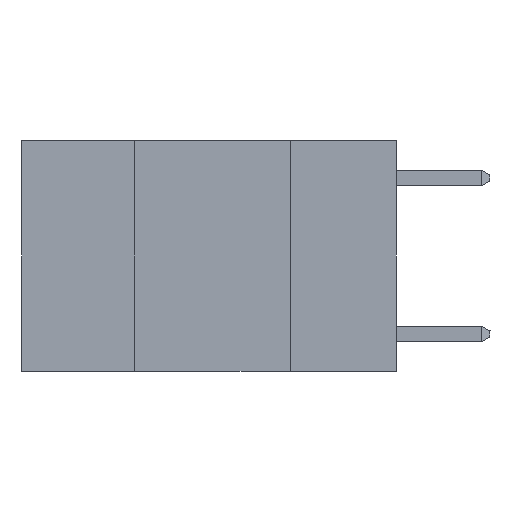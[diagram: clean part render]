
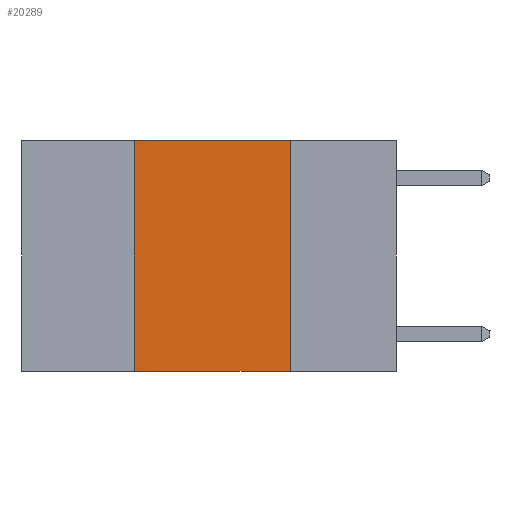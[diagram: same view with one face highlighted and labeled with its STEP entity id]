
A CAD part, left-side view. The second image highlights one B-rep face of the part: STEP entity #20289.
In plain terms, the highlighted planar face has unit normal (-1, 0, 0).
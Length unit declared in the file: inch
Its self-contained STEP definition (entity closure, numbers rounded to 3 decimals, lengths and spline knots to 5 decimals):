
#103 = VERTEX_POINT ( 'NONE', #12100 ) ;
#1859 = EDGE_CURVE ( 'NONE', #103, #26510, #22519, .T. ) ;
#2761 = AXIS2_PLACEMENT_3D ( 'NONE', #6987, #9458, #26290 ) ;
#2902 = EDGE_CURVE ( 'NONE', #11634, #26510, #29129, .T. ) ;
#4084 = DIRECTION ( 'NONE',  ( 0., 0., -1. ) ) ;
#4188 = CARTESIAN_POINT ( 'NONE',  ( 0., 0.6, -0.37 ) ) ;
#5167 = DIRECTION ( 'NONE',  ( 0., -1., 0. ) ) ;
#6987 = CARTESIAN_POINT ( 'NONE',  ( 0., 0.6, 0. ) ) ;
#7974 = CARTESIAN_POINT ( 'NONE',  ( 0., 0.42, 0. ) ) ;
#8076 = CARTESIAN_POINT ( 'NONE',  ( 0., 0.42, 0. ) ) ;
#8779 = CARTESIAN_POINT ( 'NONE',  ( 0., 0.17, 0. ) ) ;
#9458 = DIRECTION ( 'NONE',  ( 1., 0., 0. ) ) ;
#9769 = EDGE_LOOP ( 'NONE', ( #18271, #18728, #18869, #19027 ) ) ;
#11634 = VERTEX_POINT ( 'NONE', #16911 ) ;
#12100 = CARTESIAN_POINT ( 'NONE',  ( 0., 0.17, 0. ) ) ;
#12528 = CARTESIAN_POINT ( 'NONE',  ( 0., 0.6, 0. ) ) ;
#16911 = CARTESIAN_POINT ( 'NONE',  ( 0., 0.42, -0.37 ) ) ;
#16944 = CARTESIAN_POINT ( 'NONE',  ( 0., 0.17, -0.37 ) ) ;
#18271 = ORIENTED_EDGE ( 'NONE', *, *, #1859, .F. ) ;
#18728 = ORIENTED_EDGE ( 'NONE', *, *, #21424, .F. ) ;
#18869 = ORIENTED_EDGE ( 'NONE', *, *, #21526, .F. ) ;
#18950 = DIRECTION ( 'NONE',  ( 0., -1., 0. ) ) ;
#18981 = VECTOR ( 'NONE', #18950, 39.37008 ) ;
#19027 = ORIENTED_EDGE ( 'NONE', *, *, #2902, .T. ) ;
#20289 = ADVANCED_FACE ( 'NONE', ( #23175 ), #21541, .F. ) ;
#20949 = VECTOR ( 'NONE', #27339, 39.37008 ) ;
#21424 = EDGE_CURVE ( 'NONE', #21493, #103, #23890, .T. ) ;
#21493 = VERTEX_POINT ( 'NONE', #7974 ) ;
#21526 = EDGE_CURVE ( 'NONE', #11634, #21493, #27231, .T. ) ;
#21541 = PLANE ( 'NONE',  #2761 ) ;
#22220 = VECTOR ( 'NONE', #4084, 39.37008 ) ;
#22519 = LINE ( 'NONE', #8779, #22220 ) ;
#23175 = FACE_OUTER_BOUND ( 'NONE', #9769, .T. ) ;
#23890 = LINE ( 'NONE', #12528, #30182 ) ;
#26290 = DIRECTION ( 'NONE',  ( 0., 0., -1. ) ) ;
#26510 = VERTEX_POINT ( 'NONE', #16944 ) ;
#27231 = LINE ( 'NONE', #8076, #20949 ) ;
#27339 = DIRECTION ( 'NONE',  ( 0., 0., 1. ) ) ;
#29129 = LINE ( 'NONE', #4188, #18981 ) ;
#30182 = VECTOR ( 'NONE', #5167, 39.37008 ) ;
